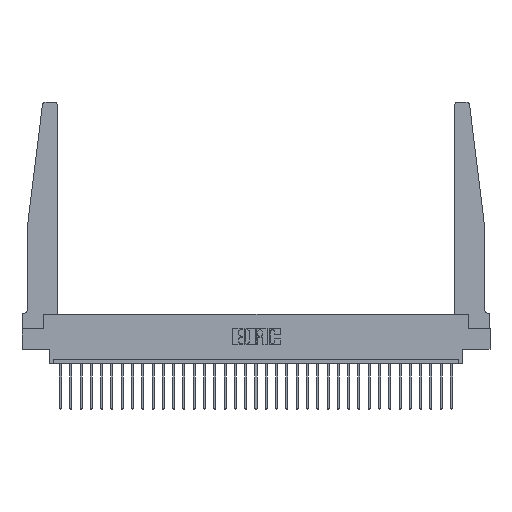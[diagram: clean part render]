
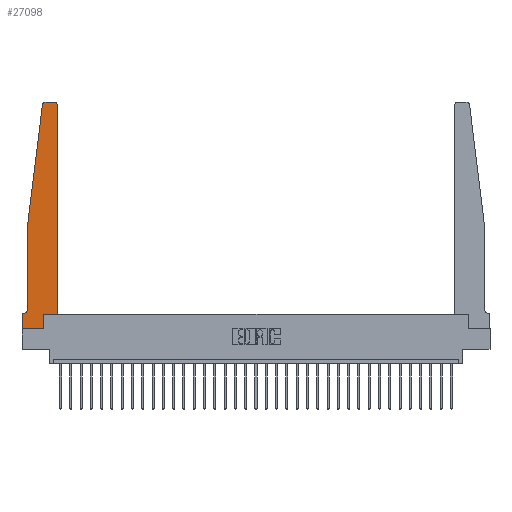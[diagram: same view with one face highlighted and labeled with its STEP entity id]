
A CAD part, top view. The second image highlights one B-rep face of the part: STEP entity #27098.
In plain terms, the highlighted planar face has unit normal (0, 0, 1).
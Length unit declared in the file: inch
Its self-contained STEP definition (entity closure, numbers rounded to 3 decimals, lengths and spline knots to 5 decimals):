
#270 = DIRECTION ( 'NONE',  ( 0., 0., 1. ) ) ;
#537 = VERTEX_POINT ( 'NONE', #3274 ) ;
#943 = EDGE_CURVE ( 'NONE', #2511, #17340, #13444, .T. ) ;
#1083 = CARTESIAN_POINT ( 'NONE',  ( 0.425, 2.72, 0.37 ) ) ;
#1157 = VERTEX_POINT ( 'NONE', #10507 ) ;
#1163 = EDGE_CURVE ( 'NONE', #10243, #13022, #15183, .T. ) ;
#1331 = EDGE_LOOP ( 'NONE', ( #20046, #10025, #6903, #26671, #2200, #9120, #22943, #17316, #8961, #23907, #2832, #8525 ) ) ;
#1432 = VECTOR ( 'NONE', #25099, 39.37008 ) ;
#1658 = AXIS2_PLACEMENT_3D ( 'NONE', #12191, #14295, #2751 ) ;
#2170 = DIRECTION ( 'NONE',  ( 0., 0., -1. ) ) ;
#2200 = ORIENTED_EDGE ( 'NONE', *, *, #6634, .T. ) ;
#2474 = CARTESIAN_POINT ( 'NONE',  ( 0., 0.1875, 0.37 ) ) ;
#2511 = VERTEX_POINT ( 'NONE', #1083 ) ;
#2712 = DIRECTION ( 'NONE',  ( 1., 0., 0. ) ) ;
#2751 = DIRECTION ( 'NONE',  ( 1., 0., 0. ) ) ;
#2832 = ORIENTED_EDGE ( 'NONE', *, *, #12299, .T. ) ;
#3274 = CARTESIAN_POINT ( 'NONE',  ( 0.065, 1.25, 0.37 ) ) ;
#3808 = AXIS2_PLACEMENT_3D ( 'NONE', #16392, #28295, #10319 ) ;
#4198 = CARTESIAN_POINT ( 'NONE',  ( 0.425, 0.18, 0.37 ) ) ;
#4388 = VERTEX_POINT ( 'NONE', #2474 ) ;
#5360 = VECTOR ( 'NONE', #8253, 39.37008 ) ;
#5517 = DIRECTION ( 'NONE',  ( -0.122, -0.992, 0. ) ) ;
#6440 = CARTESIAN_POINT ( 'NONE',  ( 0.065, 1.25, 0.37 ) ) ;
#6634 = EDGE_CURVE ( 'NONE', #21239, #28616, #19663, .T. ) ;
#6730 = VECTOR ( 'NONE', #24583, 39.37008 ) ;
#6903 = ORIENTED_EDGE ( 'NONE', *, *, #7642, .T. ) ;
#7171 = VERTEX_POINT ( 'NONE', #4198 ) ;
#7328 = EDGE_CURVE ( 'NONE', #1157, #7171, #17472, .T. ) ;
#7518 = DIRECTION ( 'NONE',  ( -1., 0., 0. ) ) ;
#7611 = CARTESIAN_POINT ( 'NONE',  ( 0.27653, 2.75, 0.37 ) ) ;
#7642 = EDGE_CURVE ( 'NONE', #13022, #537, #9330, .T. ) ;
#8253 = DIRECTION ( 'NONE',  ( 1., 0., 0. ) ) ;
#8399 = VECTOR ( 'NONE', #24503, 39.37008 ) ;
#8525 = ORIENTED_EDGE ( 'NONE', *, *, #943, .T. ) ;
#8533 = FACE_OUTER_BOUND ( 'NONE', #1331, .T. ) ;
#8961 = ORIENTED_EDGE ( 'NONE', *, *, #11260, .T. ) ;
#9120 = ORIENTED_EDGE ( 'NONE', *, *, #25818, .T. ) ;
#9330 = LINE ( 'NONE', #19268, #27766 ) ;
#9661 = CARTESIAN_POINT ( 'NONE',  ( 0.25, 2.75, 0.37 ) ) ;
#9813 = CARTESIAN_POINT ( 'NONE',  ( 0.015, 0.1875, 0.37 ) ) ;
#10025 = ORIENTED_EDGE ( 'NONE', *, *, #1163, .T. ) ;
#10243 = VERTEX_POINT ( 'NONE', #7611 ) ;
#10319 = DIRECTION ( 'NONE',  ( 1., 0., 0. ) ) ;
#10507 = CARTESIAN_POINT ( 'NONE',  ( 0.2605, 0.18, 0.37 ) ) ;
#10581 = LINE ( 'NONE', #13256, #24800 ) ;
#11260 = EDGE_CURVE ( 'NONE', #18609, #1157, #16375, .T. ) ;
#12161 = AXIS2_PLACEMENT_3D ( 'NONE', #20608, #270, #2712 ) ;
#12191 = CARTESIAN_POINT ( 'NONE',  ( 0.395, 2.72, 0.37 ) ) ;
#12299 = EDGE_CURVE ( 'NONE', #7171, #2511, #18080, .T. ) ;
#12737 = CARTESIAN_POINT ( 'NONE',  ( 0.395, 2.75, 0.37 ) ) ;
#12779 = CARTESIAN_POINT ( 'NONE',  ( 0.2605, 0., 0.37 ) ) ;
#13022 = VERTEX_POINT ( 'NONE', #20015 ) ;
#13256 = CARTESIAN_POINT ( 'NONE',  ( 0., 0., 0.37 ) ) ;
#13444 = CIRCLE ( 'NONE', #1658, 0.03 ) ;
#13507 = CARTESIAN_POINT ( 'NONE',  ( 0.015, 0.2375, 0.37 ) ) ;
#14206 = CARTESIAN_POINT ( 'NONE',  ( 0.065, 0.1875, 0.37 ) ) ;
#14295 = DIRECTION ( 'NONE',  ( 0., 0., 1. ) ) ;
#15183 = CIRCLE ( 'NONE', #12161, 0.03 ) ;
#16375 = LINE ( 'NONE', #19013, #18882 ) ;
#16392 = CARTESIAN_POINT ( 'NONE',  ( 0., 0.1875, 0.37 ) ) ;
#17316 = ORIENTED_EDGE ( 'NONE', *, *, #25857, .T. ) ;
#17340 = VERTEX_POINT ( 'NONE', #12737 ) ;
#17472 = LINE ( 'NONE', #24790, #1432 ) ;
#18080 = LINE ( 'NONE', #21977, #6730 ) ;
#18557 = LINE ( 'NONE', #26522, #5360 ) ;
#18609 = VERTEX_POINT ( 'NONE', #12779 ) ;
#18636 = EDGE_CURVE ( 'NONE', #4388, #27737, #10581, .T. ) ;
#18882 = VECTOR ( 'NONE', #29160, 39.37008 ) ;
#19013 = CARTESIAN_POINT ( 'NONE',  ( 0.2605, 0.18, 0.37 ) ) ;
#19268 = CARTESIAN_POINT ( 'NONE',  ( 0.065, 1.25, 0.37 ) ) ;
#19663 = CIRCLE ( 'NONE', #26562, 0.05 ) ;
#19971 = VECTOR ( 'NONE', #7518, 39.37008 ) ;
#20015 = CARTESIAN_POINT ( 'NONE',  ( 0.24675, 2.72367, 0.37 ) ) ;
#20046 = ORIENTED_EDGE ( 'NONE', *, *, #27930, .T. ) ;
#20608 = CARTESIAN_POINT ( 'NONE',  ( 0.27653, 2.72, 0.37 ) ) ;
#21239 = VERTEX_POINT ( 'NONE', #28121 ) ;
#21977 = CARTESIAN_POINT ( 'NONE',  ( 0.425, 0.18, 0.37 ) ) ;
#22872 = PLANE ( 'NONE',  #3808 ) ;
#22943 = ORIENTED_EDGE ( 'NONE', *, *, #18636, .T. ) ;
#23358 = VECTOR ( 'NONE', #25544, 39.37008 ) ;
#23907 = ORIENTED_EDGE ( 'NONE', *, *, #7328, .T. ) ;
#24503 = DIRECTION ( 'NONE',  ( 0., -1., 0. ) ) ;
#24583 = DIRECTION ( 'NONE',  ( 0., 1., 0. ) ) ;
#24790 = CARTESIAN_POINT ( 'NONE',  ( 0.425, 0.18, 0.37 ) ) ;
#24800 = VECTOR ( 'NONE', #26523, 39.37008 ) ;
#24971 = DIRECTION ( 'NONE',  ( -1., 0., 0. ) ) ;
#25099 = DIRECTION ( 'NONE',  ( 1., 0., 0. ) ) ;
#25544 = DIRECTION ( 'NONE',  ( -1., 0., 0. ) ) ;
#25818 = EDGE_CURVE ( 'NONE', #28616, #4388, #28159, .T. ) ;
#25857 = EDGE_CURVE ( 'NONE', #27737, #18609, #18557, .T. ) ;
#26056 = LINE ( 'NONE', #6440, #8399 ) ;
#26522 = CARTESIAN_POINT ( 'NONE',  ( 0., 0., 0.37 ) ) ;
#26523 = DIRECTION ( 'NONE',  ( 0., -1., 0. ) ) ;
#26562 = AXIS2_PLACEMENT_3D ( 'NONE', #13507, #2170, #24971 ) ;
#26671 = ORIENTED_EDGE ( 'NONE', *, *, #28374, .T. ) ;
#27098 = ADVANCED_FACE ( 'NONE', ( #8533 ), #22872, .T. ) ;
#27526 = CARTESIAN_POINT ( 'NONE',  ( 0., 0., 0.37 ) ) ;
#27737 = VERTEX_POINT ( 'NONE', #27526 ) ;
#27766 = VECTOR ( 'NONE', #5517, 39.37008 ) ;
#27930 = EDGE_CURVE ( 'NONE', #17340, #10243, #28731, .T. ) ;
#28121 = CARTESIAN_POINT ( 'NONE',  ( 0.065, 0.2375, 0.37 ) ) ;
#28159 = LINE ( 'NONE', #14206, #19971 ) ;
#28295 = DIRECTION ( 'NONE',  ( 0., 0., 1. ) ) ;
#28374 = EDGE_CURVE ( 'NONE', #537, #21239, #26056, .T. ) ;
#28616 = VERTEX_POINT ( 'NONE', #9813 ) ;
#28731 = LINE ( 'NONE', #9661, #23358 ) ;
#29160 = DIRECTION ( 'NONE',  ( 0., 1., 0. ) ) ;
